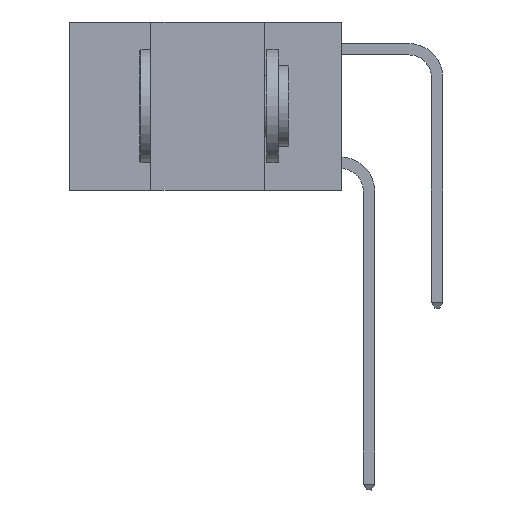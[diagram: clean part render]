
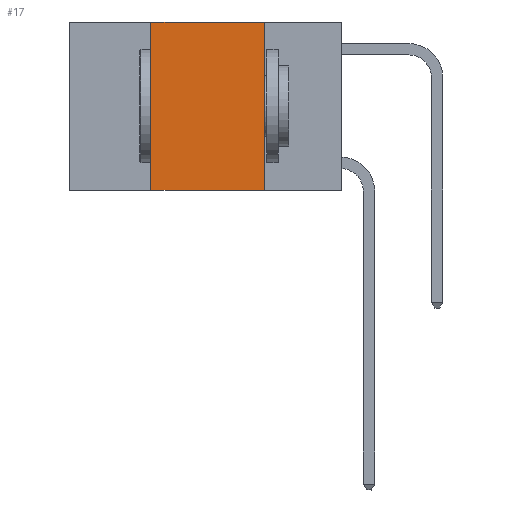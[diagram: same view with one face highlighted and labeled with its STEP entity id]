
A CAD part, left-side view. The second image highlights one B-rep face of the part: STEP entity #17.
In plain terms, the highlighted planar face has unit normal (-1, 0, 0).
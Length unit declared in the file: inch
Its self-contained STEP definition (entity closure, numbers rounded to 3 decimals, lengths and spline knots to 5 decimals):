
#17 = ADVANCED_FACE ( 'NONE', ( #5189 ), #15590, .F. ) ;
#165 = DIRECTION ( 'NONE',  ( 1., 0., 0. ) ) ;
#359 = CARTESIAN_POINT ( 'NONE',  ( 0., 0.42, 0. ) ) ;
#675 = CARTESIAN_POINT ( 'NONE',  ( 0., 0.17, -0.37 ) ) ;
#1415 = EDGE_LOOP ( 'NONE', ( #19130, #8981, #8034, #18992 ) ) ;
#1813 = DIRECTION ( 'NONE',  ( 0., 0., 1. ) ) ;
#1992 = EDGE_CURVE ( 'NONE', #17169, #14210, #9563, .T. ) ;
#2115 = CARTESIAN_POINT ( 'NONE',  ( 0., 0.6, 0. ) ) ;
#2317 = DIRECTION ( 'NONE',  ( 0., -1., 0. ) ) ;
#2602 = CARTESIAN_POINT ( 'NONE',  ( 0., 0.6, -0.37 ) ) ;
#2720 = EDGE_CURVE ( 'NONE', #14160, #14210, #3229, .T. ) ;
#3229 = LINE ( 'NONE', #4584, #5845 ) ;
#4584 = CARTESIAN_POINT ( 'NONE',  ( 0., 0.17, 0. ) ) ;
#5189 = FACE_OUTER_BOUND ( 'NONE', #1415, .T. ) ;
#5235 = EDGE_CURVE ( 'NONE', #17169, #7421, #13815, .T. ) ;
#5373 = VECTOR ( 'NONE', #1813, 39.37008 ) ;
#5845 = VECTOR ( 'NONE', #11107, 39.37008 ) ;
#7421 = VERTEX_POINT ( 'NONE', #11070 ) ;
#7459 = CARTESIAN_POINT ( 'NONE',  ( 0., 0.17, 0. ) ) ;
#8034 = ORIENTED_EDGE ( 'NONE', *, *, #5235, .F. ) ;
#8981 = ORIENTED_EDGE ( 'NONE', *, *, #13248, .F. ) ;
#9563 = LINE ( 'NONE', #2602, #15911 ) ;
#9827 = VECTOR ( 'NONE', #17993, 39.37008 ) ;
#10874 = AXIS2_PLACEMENT_3D ( 'NONE', #2115, #165, #15288 ) ;
#11070 = CARTESIAN_POINT ( 'NONE',  ( 0., 0.42, 0. ) ) ;
#11107 = DIRECTION ( 'NONE',  ( 0., 0., -1. ) ) ;
#12716 = LINE ( 'NONE', #21324, #9827 ) ;
#13248 = EDGE_CURVE ( 'NONE', #7421, #14160, #12716, .T. ) ;
#13815 = LINE ( 'NONE', #359, #5373 ) ;
#14160 = VERTEX_POINT ( 'NONE', #7459 ) ;
#14210 = VERTEX_POINT ( 'NONE', #675 ) ;
#15288 = DIRECTION ( 'NONE',  ( 0., 0., -1. ) ) ;
#15590 = PLANE ( 'NONE',  #10874 ) ;
#15911 = VECTOR ( 'NONE', #2317, 39.37008 ) ;
#16221 = CARTESIAN_POINT ( 'NONE',  ( 0., 0.42, -0.37 ) ) ;
#17169 = VERTEX_POINT ( 'NONE', #16221 ) ;
#17993 = DIRECTION ( 'NONE',  ( 0., -1., 0. ) ) ;
#18992 = ORIENTED_EDGE ( 'NONE', *, *, #1992, .T. ) ;
#19130 = ORIENTED_EDGE ( 'NONE', *, *, #2720, .F. ) ;
#21324 = CARTESIAN_POINT ( 'NONE',  ( 0., 0.6, 0. ) ) ;
